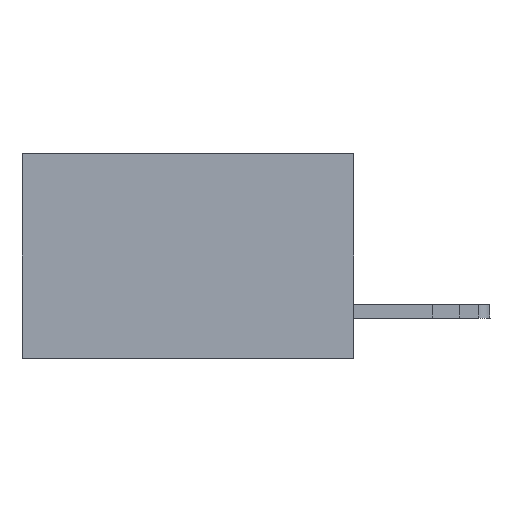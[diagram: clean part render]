
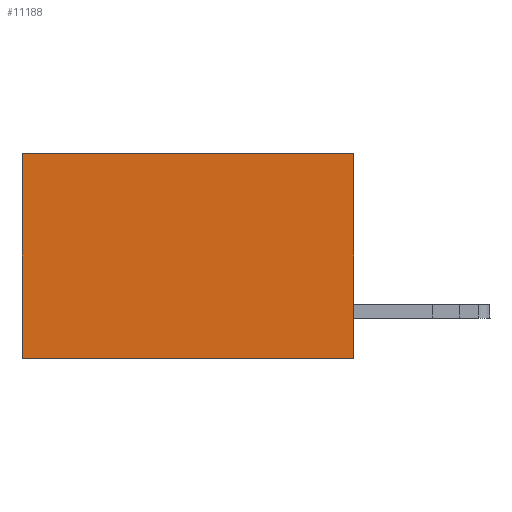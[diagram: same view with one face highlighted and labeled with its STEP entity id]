
A CAD part, left-side view. The second image highlights one B-rep face of the part: STEP entity #11188.
In plain terms, the highlighted planar face has unit normal (-1, 0, 0).
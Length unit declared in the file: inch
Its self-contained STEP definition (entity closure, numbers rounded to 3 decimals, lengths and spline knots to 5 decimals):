
#3180 = EDGE_CURVE ( 'NONE', #25507, #6503, #7332, .T. ) ;
#3490 = DIRECTION ( 'NONE',  ( 0., 0., -1. ) ) ;
#4433 = CARTESIAN_POINT ( 'NONE',  ( 0.2875, 0., -0.37 ) ) ;
#4566 = DIRECTION ( 'NONE',  ( 0., 1., 0. ) ) ;
#5637 = PLANE ( 'NONE',  #13831 ) ;
#6067 = VECTOR ( 'NONE', #3490, 39.37008 ) ;
#6503 = VERTEX_POINT ( 'NONE', #10884 ) ;
#6777 = LINE ( 'NONE', #25779, #6067 ) ;
#6895 = VECTOR ( 'NONE', #18769, 39.37008 ) ;
#6984 = VERTEX_POINT ( 'NONE', #26483 ) ;
#7332 = LINE ( 'NONE', #17020, #24763 ) ;
#8780 = LINE ( 'NONE', #24503, #27928 ) ;
#9019 = EDGE_LOOP ( 'NONE', ( #28465, #25670, #18298, #21884 ) ) ;
#10884 = CARTESIAN_POINT ( 'NONE',  ( 0.2875, 0.6, -0.37 ) ) ;
#11183 = EDGE_CURVE ( 'NONE', #6984, #11991, #6777, .T. ) ;
#11188 = ADVANCED_FACE ( 'NONE', ( #13498 ), #5637, .F. ) ;
#11991 = VERTEX_POINT ( 'NONE', #4433 ) ;
#12358 = DIRECTION ( 'NONE',  ( 0., 0., -1. ) ) ;
#13024 = EDGE_CURVE ( 'NONE', #6984, #25507, #8780, .T. ) ;
#13498 = FACE_OUTER_BOUND ( 'NONE', #9019, .T. ) ;
#13831 = AXIS2_PLACEMENT_3D ( 'NONE', #23562, #19307, #23458 ) ;
#14114 = CARTESIAN_POINT ( 'NONE',  ( 0.2875, 0.6, 0. ) ) ;
#15653 = CARTESIAN_POINT ( 'NONE',  ( 0.2875, 0., -0.37 ) ) ;
#17020 = CARTESIAN_POINT ( 'NONE',  ( 0.2875, 0.6, 0. ) ) ;
#18298 = ORIENTED_EDGE ( 'NONE', *, *, #11183, .F. ) ;
#18769 = DIRECTION ( 'NONE',  ( 0., 1., 0. ) ) ;
#19307 = DIRECTION ( 'NONE',  ( 1., 0., 0. ) ) ;
#21884 = ORIENTED_EDGE ( 'NONE', *, *, #13024, .T. ) ;
#23458 = DIRECTION ( 'NONE',  ( 0., 0., -1. ) ) ;
#23562 = CARTESIAN_POINT ( 'NONE',  ( 0.2875, 0., 0. ) ) ;
#24205 = EDGE_CURVE ( 'NONE', #11991, #6503, #26052, .T. ) ;
#24503 = CARTESIAN_POINT ( 'NONE',  ( 0.2875, 0., 0. ) ) ;
#24763 = VECTOR ( 'NONE', #12358, 39.37008 ) ;
#25507 = VERTEX_POINT ( 'NONE', #14114 ) ;
#25670 = ORIENTED_EDGE ( 'NONE', *, *, #24205, .F. ) ;
#25779 = CARTESIAN_POINT ( 'NONE',  ( 0.2875, 0., 0. ) ) ;
#26052 = LINE ( 'NONE', #15653, #6895 ) ;
#26483 = CARTESIAN_POINT ( 'NONE',  ( 0.2875, 0., 0. ) ) ;
#27928 = VECTOR ( 'NONE', #4566, 39.37008 ) ;
#28465 = ORIENTED_EDGE ( 'NONE', *, *, #3180, .T. ) ;
